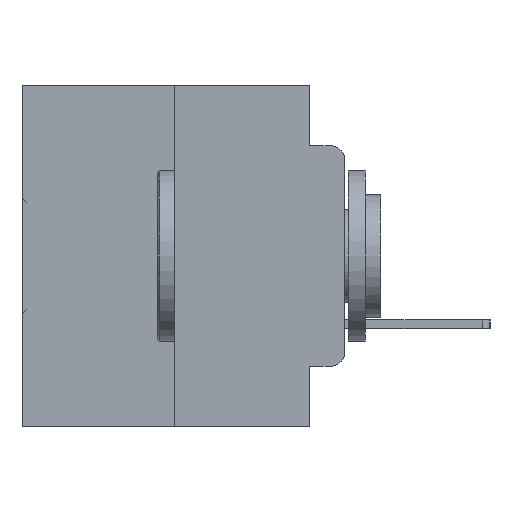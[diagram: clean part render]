
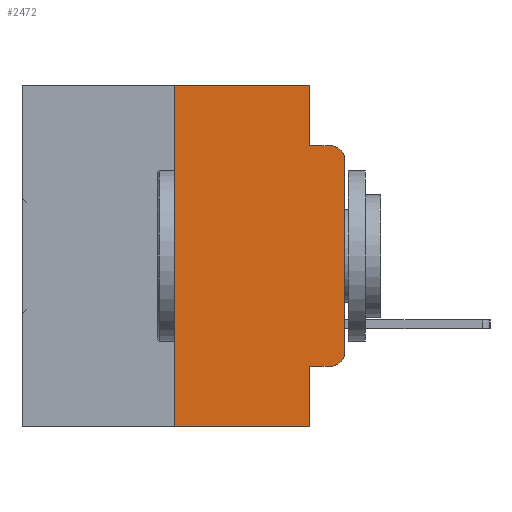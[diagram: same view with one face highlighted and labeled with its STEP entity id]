
A CAD part, left-side view. The second image highlights one B-rep face of the part: STEP entity #2472.
In plain terms, the highlighted planar face has unit normal (-1, 0, 0).
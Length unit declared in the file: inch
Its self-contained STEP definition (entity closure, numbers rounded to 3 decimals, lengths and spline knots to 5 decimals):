
#626 = CARTESIAN_POINT ( 'NONE',  ( 0., 0., 0. ) ) ;
#837 = VERTEX_POINT ( 'NONE', #27042 ) ;
#1161 = AXIS2_PLACEMENT_3D ( 'NONE', #32553, #24705, #3716 ) ;
#1256 = LINE ( 'NONE', #10428, #27435 ) ;
#2099 = VERTEX_POINT ( 'NONE', #30728 ) ;
#2472 = ADVANCED_FACE ( 'NONE', ( #7892 ), #20777, .F. ) ;
#3359 = DIRECTION ( 'NONE',  ( 0., -1., 0. ) ) ;
#3480 = CARTESIAN_POINT ( 'NONE',  ( 0., 0.051, 0. ) ) ;
#3513 = ORIENTED_EDGE ( 'NONE', *, *, #10979, .F. ) ;
#3598 = VECTOR ( 'NONE', #18984, 39.37008 ) ;
#3716 = DIRECTION ( 'NONE',  ( 0., 0., -1. ) ) ;
#3801 = LINE ( 'NONE', #24339, #30740 ) ;
#4031 = CARTESIAN_POINT ( 'NONE',  ( 0., 0.25, -0.5 ) ) ;
#4783 = CARTESIAN_POINT ( 'NONE',  ( 0., 0.25, 0. ) ) ;
#5104 = CARTESIAN_POINT ( 'NONE',  ( 0., 0.02, -0.0885 ) ) ;
#5270 = CIRCLE ( 'NONE', #20489, 0.02 ) ;
#6172 = CARTESIAN_POINT ( 'NONE',  ( 0., 0.051, 0. ) ) ;
#6955 = VECTOR ( 'NONE', #3359, 39.37008 ) ;
#7880 = EDGE_CURVE ( 'NONE', #31476, #12358, #30903, .T. ) ;
#7892 = FACE_OUTER_BOUND ( 'NONE', #15777, .T. ) ;
#8198 = CARTESIAN_POINT ( 'NONE',  ( 0., 0.02, -0.1085 ) ) ;
#8469 = AXIS2_PLACEMENT_3D ( 'NONE', #8198, #26400, #10868 ) ;
#8500 = ORIENTED_EDGE ( 'NONE', *, *, #9443, .F. ) ;
#8737 = DIRECTION ( 'NONE',  ( 0., -1., 0. ) ) ;
#9086 = VERTEX_POINT ( 'NONE', #6172 ) ;
#9215 = CARTESIAN_POINT ( 'NONE',  ( 0., 0.02, -0.3915 ) ) ;
#9443 = EDGE_CURVE ( 'NONE', #24508, #22598, #1256, .T. ) ;
#9769 = CARTESIAN_POINT ( 'NONE',  ( 0., 0.051, -0.0885 ) ) ;
#10064 = EDGE_CURVE ( 'NONE', #837, #19105, #33878, .T. ) ;
#10428 = CARTESIAN_POINT ( 'NONE',  ( 0., 0.051, 0. ) ) ;
#10472 = ORIENTED_EDGE ( 'NONE', *, *, #20704, .T. ) ;
#10868 = DIRECTION ( 'NONE',  ( 0., 0., -1. ) ) ;
#10979 = EDGE_CURVE ( 'NONE', #12358, #9086, #19991, .T. ) ;
#11014 = VECTOR ( 'NONE', #32654, 39.37008 ) ;
#11135 = CARTESIAN_POINT ( 'NONE',  ( 0., 0.473, -0.5 ) ) ;
#11329 = CARTESIAN_POINT ( 'NONE',  ( 0., 0.473, 0. ) ) ;
#11476 = EDGE_CURVE ( 'NONE', #33792, #30812, #5270, .T. ) ;
#11889 = DIRECTION ( 'NONE',  ( 0., 0., -1. ) ) ;
#12056 = CARTESIAN_POINT ( 'NONE',  ( 0., 0., -0.3915 ) ) ;
#12358 = VERTEX_POINT ( 'NONE', #4783 ) ;
#13799 = DIRECTION ( 'NONE',  ( 0., -1., 0. ) ) ;
#14299 = ORIENTED_EDGE ( 'NONE', *, *, #29489, .T. ) ;
#15777 = EDGE_LOOP ( 'NONE', ( #10472, #30805, #18248, #24776, #3513, #17902, #32500, #8500, #14299, #21946 ) ) ;
#15993 = VECTOR ( 'NONE', #27000, 39.37008 ) ;
#16370 = EDGE_CURVE ( 'NONE', #31476, #22598, #22903, .T. ) ;
#16829 = VECTOR ( 'NONE', #13799, 39.37008 ) ;
#17615 = LINE ( 'NONE', #3480, #15993 ) ;
#17902 = ORIENTED_EDGE ( 'NONE', *, *, #7880, .F. ) ;
#18248 = ORIENTED_EDGE ( 'NONE', *, *, #10064, .F. ) ;
#18984 = DIRECTION ( 'NONE',  ( 0., 0., 1. ) ) ;
#19105 = VERTEX_POINT ( 'NONE', #5104 ) ;
#19160 = CIRCLE ( 'NONE', #8469, 0.02 ) ;
#19707 = CARTESIAN_POINT ( 'NONE',  ( 0., 0.25, 0. ) ) ;
#19991 = LINE ( 'NONE', #11329, #6955 ) ;
#20489 = AXIS2_PLACEMENT_3D ( 'NONE', #9215, #27407, #11889 ) ;
#20704 = EDGE_CURVE ( 'NONE', #30812, #2099, #24457, .T. ) ;
#20777 = PLANE ( 'NONE',  #1161 ) ;
#21946 = ORIENTED_EDGE ( 'NONE', *, *, #11476, .T. ) ;
#22598 = VERTEX_POINT ( 'NONE', #26518 ) ;
#22903 = LINE ( 'NONE', #11135, #16829 ) ;
#24339 = CARTESIAN_POINT ( 'NONE',  ( 0., 0.051, -0.4115 ) ) ;
#24457 = LINE ( 'NONE', #626, #3598 ) ;
#24508 = VERTEX_POINT ( 'NONE', #29237 ) ;
#24705 = DIRECTION ( 'NONE',  ( 1., 0., 0. ) ) ;
#24776 = ORIENTED_EDGE ( 'NONE', *, *, #32679, .F. ) ;
#25242 = CARTESIAN_POINT ( 'NONE',  ( 0., 0.02, -0.4115 ) ) ;
#26400 = DIRECTION ( 'NONE',  ( -1., 0., 0. ) ) ;
#26518 = CARTESIAN_POINT ( 'NONE',  ( 0., 0.051, -0.5 ) ) ;
#26576 = EDGE_CURVE ( 'NONE', #2099, #19105, #19160, .T. ) ;
#27000 = DIRECTION ( 'NONE',  ( 0., 0., -1. ) ) ;
#27042 = CARTESIAN_POINT ( 'NONE',  ( 0., 0.051, -0.0885 ) ) ;
#27407 = DIRECTION ( 'NONE',  ( -1., 0., 0. ) ) ;
#27435 = VECTOR ( 'NONE', #29543, 39.37008 ) ;
#27935 = DIRECTION ( 'NONE',  ( 0., -1., 0. ) ) ;
#29237 = CARTESIAN_POINT ( 'NONE',  ( 0., 0.051, -0.4115 ) ) ;
#29489 = EDGE_CURVE ( 'NONE', #24508, #33792, #3801, .T. ) ;
#29543 = DIRECTION ( 'NONE',  ( 0., 0., -1. ) ) ;
#30728 = CARTESIAN_POINT ( 'NONE',  ( 0., 0., -0.1085 ) ) ;
#30740 = VECTOR ( 'NONE', #8737, 39.37008 ) ;
#30805 = ORIENTED_EDGE ( 'NONE', *, *, #26576, .T. ) ;
#30812 = VERTEX_POINT ( 'NONE', #12056 ) ;
#30903 = LINE ( 'NONE', #19707, #11014 ) ;
#31476 = VERTEX_POINT ( 'NONE', #4031 ) ;
#32500 = ORIENTED_EDGE ( 'NONE', *, *, #16370, .T. ) ;
#32553 = CARTESIAN_POINT ( 'NONE',  ( 0., 0.473, 0. ) ) ;
#32654 = DIRECTION ( 'NONE',  ( 0., 0., 1. ) ) ;
#32679 = EDGE_CURVE ( 'NONE', #9086, #837, #17615, .T. ) ;
#33050 = VECTOR ( 'NONE', #27935, 39.37008 ) ;
#33792 = VERTEX_POINT ( 'NONE', #25242 ) ;
#33878 = LINE ( 'NONE', #9769, #33050 ) ;
